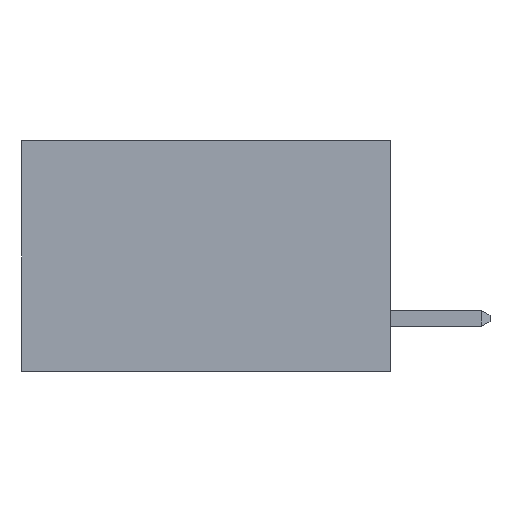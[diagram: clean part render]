
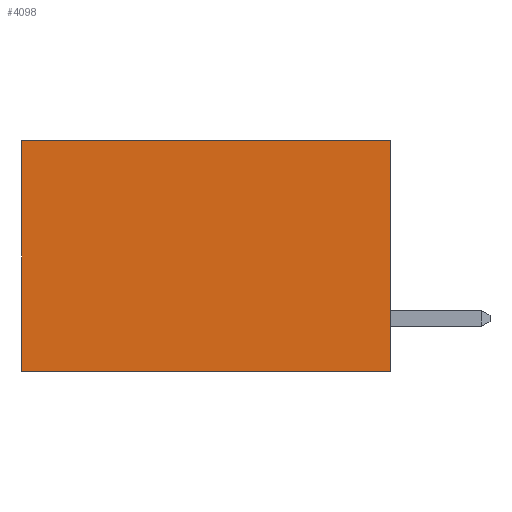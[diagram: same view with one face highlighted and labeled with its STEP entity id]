
A CAD part, left-side view. The second image highlights one B-rep face of the part: STEP entity #4098.
In plain terms, the highlighted planar face has unit normal (-1, 0, 0).
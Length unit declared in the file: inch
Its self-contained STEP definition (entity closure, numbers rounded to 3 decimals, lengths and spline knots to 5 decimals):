
#285 = VERTEX_POINT ( 'NONE', #10483 ) ;
#311 = EDGE_CURVE ( 'NONE', #13258, #285, #5855, .T. ) ;
#1499 = EDGE_CURVE ( 'NONE', #14111, #19168, #11535, .T. ) ;
#1817 = DIRECTION ( 'NONE',  ( 0., 0., -1. ) ) ;
#3509 = ORIENTED_EDGE ( 'NONE', *, *, #7096, .F. ) ;
#3749 = CARTESIAN_POINT ( 'NONE',  ( 0.277, 0.59, -0.37 ) ) ;
#3883 = FACE_OUTER_BOUND ( 'NONE', #11783, .T. ) ;
#4000 = CARTESIAN_POINT ( 'NONE',  ( 0.277, 0., -0.37 ) ) ;
#4098 = ADVANCED_FACE ( 'NONE', ( #3883 ), #12671, .F. ) ;
#5855 = LINE ( 'NONE', #10383, #15485 ) ;
#6410 = VECTOR ( 'NONE', #24532, 39.37008 ) ;
#7096 = EDGE_CURVE ( 'NONE', #13258, #14111, #23461, .T. ) ;
#8350 = CARTESIAN_POINT ( 'NONE',  ( 0.277, 0.59, -0.37 ) ) ;
#9009 = EDGE_CURVE ( 'NONE', #285, #19168, #24587, .T. ) ;
#10383 = CARTESIAN_POINT ( 'NONE',  ( 0.277, 0., 0. ) ) ;
#10483 = CARTESIAN_POINT ( 'NONE',  ( 0.277, 0.59, 0. ) ) ;
#11121 = ORIENTED_EDGE ( 'NONE', *, *, #1499, .F. ) ;
#11535 = LINE ( 'NONE', #22397, #6410 ) ;
#11783 = EDGE_LOOP ( 'NONE', ( #17033, #11121, #3509, #16843 ) ) ;
#12116 = CARTESIAN_POINT ( 'NONE',  ( 0.277, 0., 0. ) ) ;
#12485 = DIRECTION ( 'NONE',  ( 0., 0., -1. ) ) ;
#12560 = DIRECTION ( 'NONE',  ( 1., 0., 0. ) ) ;
#12671 = PLANE ( 'NONE',  #18479 ) ;
#13258 = VERTEX_POINT ( 'NONE', #12116 ) ;
#13957 = CARTESIAN_POINT ( 'NONE',  ( 0.277, 0., -0.37 ) ) ;
#14111 = VERTEX_POINT ( 'NONE', #16364 ) ;
#15485 = VECTOR ( 'NONE', #24298, 39.37008 ) ;
#16364 = CARTESIAN_POINT ( 'NONE',  ( 0.277, 0., -0.37 ) ) ;
#16843 = ORIENTED_EDGE ( 'NONE', *, *, #311, .T. ) ;
#17033 = ORIENTED_EDGE ( 'NONE', *, *, #9009, .T. ) ;
#18479 = AXIS2_PLACEMENT_3D ( 'NONE', #13957, #12560, #12485 ) ;
#18951 = VECTOR ( 'NONE', #1817, 39.37008 ) ;
#19168 = VERTEX_POINT ( 'NONE', #8350 ) ;
#19359 = DIRECTION ( 'NONE',  ( 0., 0., -1. ) ) ;
#22397 = CARTESIAN_POINT ( 'NONE',  ( 0.277, 0., -0.37 ) ) ;
#22882 = VECTOR ( 'NONE', #19359, 39.37008 ) ;
#23461 = LINE ( 'NONE', #4000, #22882 ) ;
#24298 = DIRECTION ( 'NONE',  ( 0., 1., 0. ) ) ;
#24532 = DIRECTION ( 'NONE',  ( 0., 1., 0. ) ) ;
#24587 = LINE ( 'NONE', #3749, #18951 ) ;
